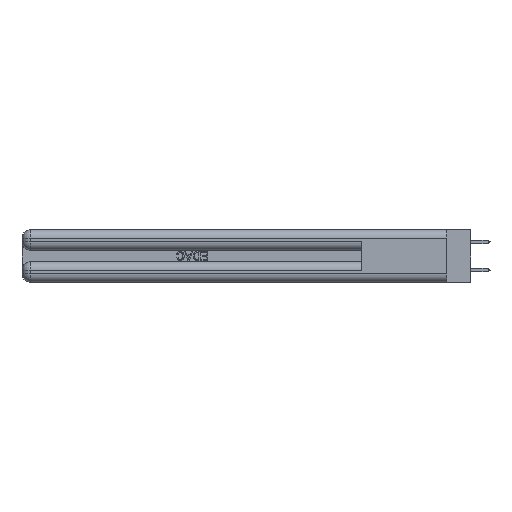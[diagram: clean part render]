
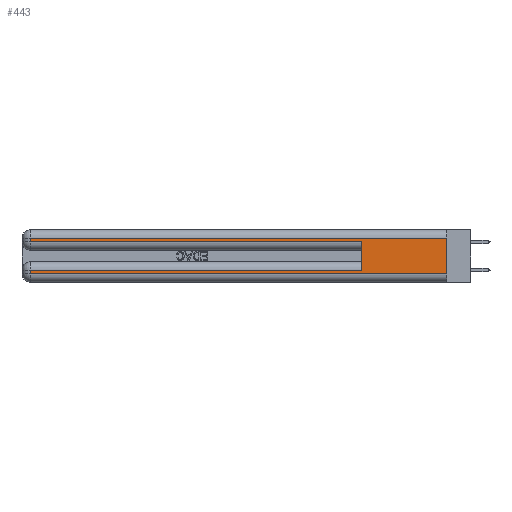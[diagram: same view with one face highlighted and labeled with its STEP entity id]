
A CAD part, left-side view. The second image highlights one B-rep face of the part: STEP entity #443.
In plain terms, the highlighted planar face has unit normal (-1, 0, 0).
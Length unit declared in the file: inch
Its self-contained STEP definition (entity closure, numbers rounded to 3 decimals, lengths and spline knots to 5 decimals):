
#8 = FACE_OUTER_BOUND ( 'NONE', #42237, .T. ) ;
#82 = ORIENTED_EDGE ( 'NONE', *, *, #38951, .T. ) ;
#157 = EDGE_CURVE ( 'NONE', #19381, #11633, #36222, .T. ) ;
#396 = VECTOR ( 'NONE', #18739, 39.37008 ) ;
#443 = ADVANCED_FACE ( 'NONE', ( #8 ), #39309, .F. ) ;
#861 = LINE ( 'NONE', #25841, #4251 ) ;
#927 = VERTEX_POINT ( 'NONE', #38281 ) ;
#2304 = EDGE_CURVE ( 'NONE', #22369, #927, #32259, .T. ) ;
#2644 = DIRECTION ( 'NONE',  ( 0., 0., -1. ) ) ;
#3484 = DIRECTION ( 'NONE',  ( 1., 0., 0. ) ) ;
#3868 = VERTEX_POINT ( 'NONE', #31571 ) ;
#3925 = LINE ( 'NONE', #27481, #31299 ) ;
#4066 = CARTESIAN_POINT ( 'NONE',  ( 0., 0., 0.285 ) ) ;
#4251 = VECTOR ( 'NONE', #29872, 39.37008 ) ;
#4504 = CARTESIAN_POINT ( 'NONE',  ( 0., 0., 0.06 ) ) ;
#7575 = ORIENTED_EDGE ( 'NONE', *, *, #2304, .T. ) ;
#7647 = LINE ( 'NONE', #4504, #396 ) ;
#9775 = CARTESIAN_POINT ( 'NONE',  ( 0., 0., 0.06 ) ) ;
#10160 = CARTESIAN_POINT ( 'NONE',  ( 0., 2.94, 0.31 ) ) ;
#11633 = VERTEX_POINT ( 'NONE', #10160 ) ;
#11791 = ORIENTED_EDGE ( 'NONE', *, *, #25745, .T. ) ;
#13158 = LINE ( 'NONE', #39318, #41565 ) ;
#13522 = ORIENTED_EDGE ( 'NONE', *, *, #43955, .T. ) ;
#17171 = CARTESIAN_POINT ( 'NONE',  ( 0., 0., 0.085 ) ) ;
#18513 = CARTESIAN_POINT ( 'NONE',  ( 0., 2.94, 0.085 ) ) ;
#18739 = DIRECTION ( 'NONE',  ( 0., -1., 0. ) ) ;
#19126 = VERTEX_POINT ( 'NONE', #18513 ) ;
#19140 = ORIENTED_EDGE ( 'NONE', *, *, #19368, .F. ) ;
#19368 = EDGE_CURVE ( 'NONE', #19381, #30307, #861, .T. ) ;
#19381 = VERTEX_POINT ( 'NONE', #22768 ) ;
#20823 = ORIENTED_EDGE ( 'NONE', *, *, #40595, .F. ) ;
#22369 = VERTEX_POINT ( 'NONE', #25922 ) ;
#22483 = LINE ( 'NONE', #44638, #44736 ) ;
#22768 = CARTESIAN_POINT ( 'NONE',  ( 0., 0., 0.31 ) ) ;
#24198 = DIRECTION ( 'NONE',  ( 0., 1., 0. ) ) ;
#25309 = VERTEX_POINT ( 'NONE', #45714 ) ;
#25745 = EDGE_CURVE ( 'NONE', #25309, #19126, #37389, .T. ) ;
#25841 = CARTESIAN_POINT ( 'NONE',  ( 0., 0., 0.37 ) ) ;
#25922 = CARTESIAN_POINT ( 'NONE',  ( 0., 2.94, 0.285 ) ) ;
#26260 = VECTOR ( 'NONE', #24198, 39.37008 ) ;
#27481 = CARTESIAN_POINT ( 'NONE',  ( 0., 2.94, 0.37 ) ) ;
#29872 = DIRECTION ( 'NONE',  ( 0., 0., -1. ) ) ;
#30307 = VERTEX_POINT ( 'NONE', #9775 ) ;
#31299 = VECTOR ( 'NONE', #2644, 39.37008 ) ;
#31571 = CARTESIAN_POINT ( 'NONE',  ( 0., 2.94, 0.06 ) ) ;
#32012 = CARTESIAN_POINT ( 'NONE',  ( 0., 0., 0.37 ) ) ;
#32259 = LINE ( 'NONE', #4066, #44514 ) ;
#33075 = ORIENTED_EDGE ( 'NONE', *, *, #36075, .T. ) ;
#35302 = DIRECTION ( 'NONE',  ( 0., 0., -1. ) ) ;
#35627 = DIRECTION ( 'NONE',  ( 0., 1., 0. ) ) ;
#36075 = EDGE_CURVE ( 'NONE', #11633, #22369, #3925, .T. ) ;
#36222 = LINE ( 'NONE', #41752, #26260 ) ;
#37389 = LINE ( 'NONE', #17171, #44026 ) ;
#38131 = ORIENTED_EDGE ( 'NONE', *, *, #157, .T. ) ;
#38281 = CARTESIAN_POINT ( 'NONE',  ( 0., 0.6, 0.285 ) ) ;
#38951 = EDGE_CURVE ( 'NONE', #19126, #3868, #13158, .T. ) ;
#39309 = PLANE ( 'NONE',  #45887 ) ;
#39318 = CARTESIAN_POINT ( 'NONE',  ( 0., 2.94, 0.37 ) ) ;
#40595 = EDGE_CURVE ( 'NONE', #25309, #927, #22483, .T. ) ;
#41525 = DIRECTION ( 'NONE',  ( 0., 0., 1. ) ) ;
#41565 = VECTOR ( 'NONE', #46024, 39.37008 ) ;
#41752 = CARTESIAN_POINT ( 'NONE',  ( 0., 0., 0.31 ) ) ;
#42237 = EDGE_LOOP ( 'NONE', ( #19140, #38131, #33075, #7575, #20823, #11791, #82, #13522 ) ) ;
#42883 = DIRECTION ( 'NONE',  ( 0., -1., 0. ) ) ;
#43955 = EDGE_CURVE ( 'NONE', #3868, #30307, #7647, .T. ) ;
#44026 = VECTOR ( 'NONE', #35627, 39.37008 ) ;
#44514 = VECTOR ( 'NONE', #42883, 39.37008 ) ;
#44638 = CARTESIAN_POINT ( 'NONE',  ( 0., 0.6, 0.145 ) ) ;
#44736 = VECTOR ( 'NONE', #41525, 39.37008 ) ;
#45714 = CARTESIAN_POINT ( 'NONE',  ( 0., 0.6, 0.085 ) ) ;
#45887 = AXIS2_PLACEMENT_3D ( 'NONE', #32012, #3484, #35302 ) ;
#46024 = DIRECTION ( 'NONE',  ( 0., 0., -1. ) ) ;
